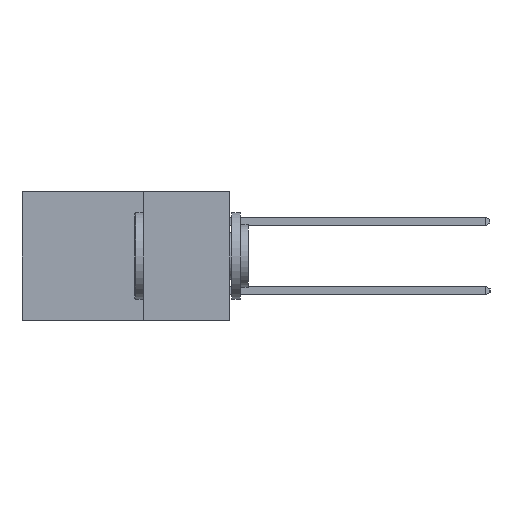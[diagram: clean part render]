
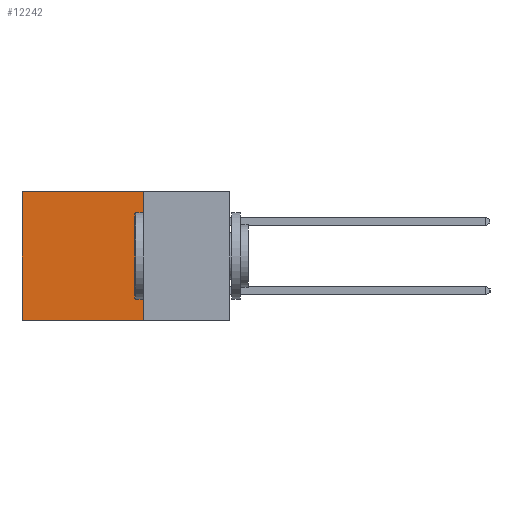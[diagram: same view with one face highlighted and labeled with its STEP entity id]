
A CAD part, left-side view. The second image highlights one B-rep face of the part: STEP entity #12242.
In plain terms, the highlighted planar face has unit normal (-1, 0, 0).
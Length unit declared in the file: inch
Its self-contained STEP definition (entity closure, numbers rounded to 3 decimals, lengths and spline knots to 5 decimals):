
#761 = VERTEX_POINT ( 'NONE', #1778 ) ;
#917 = LINE ( 'NONE', #2740, #12123 ) ;
#1296 = CARTESIAN_POINT ( 'NONE',  ( 0.2615, 0.25, -0.37 ) ) ;
#1778 = CARTESIAN_POINT ( 'NONE',  ( 0.2615, 0.6, 0. ) ) ;
#1783 = PLANE ( 'NONE',  #13808 ) ;
#2062 = ORIENTED_EDGE ( 'NONE', *, *, #12263, .F. ) ;
#2295 = VECTOR ( 'NONE', #4490, 39.37008 ) ;
#2603 = CARTESIAN_POINT ( 'NONE',  ( 0.2615, 0.25, 0. ) ) ;
#2725 = DIRECTION ( 'NONE',  ( 0., 1., 0. ) ) ;
#2740 = CARTESIAN_POINT ( 'NONE',  ( 0.2615, 0.25, -0.37 ) ) ;
#2942 = DIRECTION ( 'NONE',  ( 1., 0., 0. ) ) ;
#2998 = DIRECTION ( 'NONE',  ( 0., 0., -1. ) ) ;
#3798 = DIRECTION ( 'NONE',  ( 0., 1., 0. ) ) ;
#3866 = CARTESIAN_POINT ( 'NONE',  ( 0.2615, 0.25, 0. ) ) ;
#4406 = EDGE_CURVE ( 'NONE', #761, #9882, #14086, .T. ) ;
#4490 = DIRECTION ( 'NONE',  ( 0., 0., -1. ) ) ;
#4530 = CARTESIAN_POINT ( 'NONE',  ( 0.2615, 0.6, -0.37 ) ) ;
#4545 = EDGE_CURVE ( 'NONE', #12632, #9882, #917, .T. ) ;
#5235 = CARTESIAN_POINT ( 'NONE',  ( 0.2615, 0.25, -0.37 ) ) ;
#6166 = VERTEX_POINT ( 'NONE', #2603 ) ;
#6360 = ORIENTED_EDGE ( 'NONE', *, *, #4406, .T. ) ;
#6977 = ORIENTED_EDGE ( 'NONE', *, *, #8231, .T. ) ;
#8231 = EDGE_CURVE ( 'NONE', #6166, #761, #9366, .T. ) ;
#9343 = ORIENTED_EDGE ( 'NONE', *, *, #4545, .F. ) ;
#9366 = LINE ( 'NONE', #3866, #11883 ) ;
#9882 = VERTEX_POINT ( 'NONE', #11377 ) ;
#10131 = EDGE_LOOP ( 'NONE', ( #6360, #9343, #2062, #6977 ) ) ;
#10726 = VECTOR ( 'NONE', #2998, 39.37008 ) ;
#10818 = DIRECTION ( 'NONE',  ( 0., 0., -1. ) ) ;
#11377 = CARTESIAN_POINT ( 'NONE',  ( 0.2615, 0.6, -0.37 ) ) ;
#11397 = LINE ( 'NONE', #11942, #10726 ) ;
#11883 = VECTOR ( 'NONE', #3798, 39.37008 ) ;
#11942 = CARTESIAN_POINT ( 'NONE',  ( 0.2615, 0.25, -0.37 ) ) ;
#12123 = VECTOR ( 'NONE', #2725, 39.37008 ) ;
#12242 = ADVANCED_FACE ( 'NONE', ( #13878 ), #1783, .F. ) ;
#12263 = EDGE_CURVE ( 'NONE', #6166, #12632, #11397, .T. ) ;
#12632 = VERTEX_POINT ( 'NONE', #1296 ) ;
#13808 = AXIS2_PLACEMENT_3D ( 'NONE', #5235, #2942, #10818 ) ;
#13878 = FACE_OUTER_BOUND ( 'NONE', #10131, .T. ) ;
#14086 = LINE ( 'NONE', #4530, #2295 ) ;
